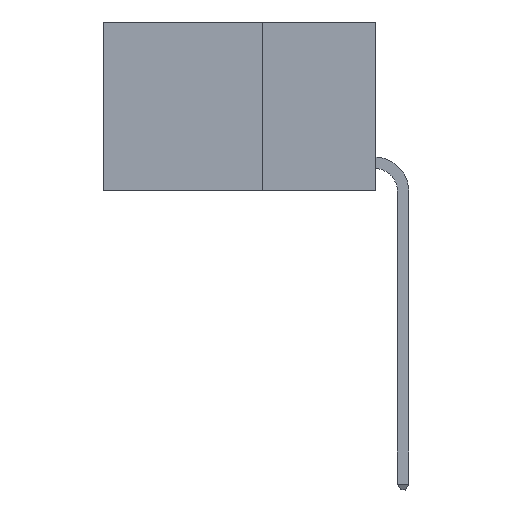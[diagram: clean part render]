
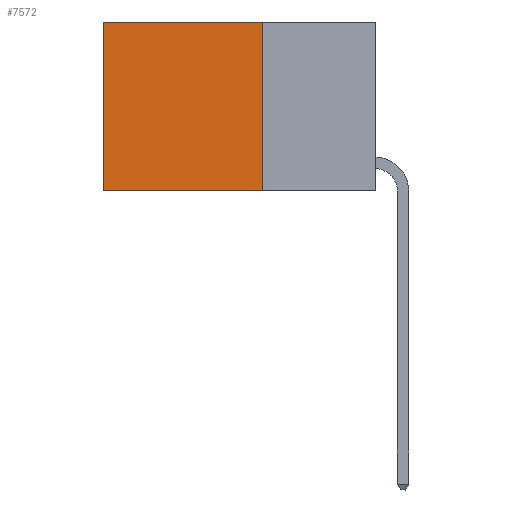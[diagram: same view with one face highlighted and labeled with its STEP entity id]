
A CAD part, left-side view. The second image highlights one B-rep face of the part: STEP entity #7572.
In plain terms, the highlighted planar face has unit normal (-1, 0, 0).
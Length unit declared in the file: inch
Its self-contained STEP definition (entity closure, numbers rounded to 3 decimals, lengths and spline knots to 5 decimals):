
#388 = ORIENTED_EDGE ( 'NONE', *, *, #1872, .F. ) ;
#816 = ORIENTED_EDGE ( 'NONE', *, *, #11375, .F. ) ;
#940 = EDGE_LOOP ( 'NONE', ( #3710, #388, #816, #11710 ) ) ;
#1307 = DIRECTION ( 'NONE',  ( 0., 1., 0. ) ) ;
#1872 = EDGE_CURVE ( 'NONE', #12418, #19040, #2484, .T. ) ;
#2484 = LINE ( 'NONE', #6540, #23468 ) ;
#2777 = VECTOR ( 'NONE', #6769, 39.37008 ) ;
#3455 = VECTOR ( 'NONE', #1307, 39.37008 ) ;
#3710 = ORIENTED_EDGE ( 'NONE', *, *, #16071, .T. ) ;
#3815 = VECTOR ( 'NONE', #17820, 39.37008 ) ;
#3873 = DIRECTION ( 'NONE',  ( 1., 0., 0. ) ) ;
#5211 = AXIS2_PLACEMENT_3D ( 'NONE', #17115, #3873, #11581 ) ;
#5251 = CARTESIAN_POINT ( 'NONE',  ( 0.2625, 0.25, 0. ) ) ;
#5885 = PLANE ( 'NONE',  #5211 ) ;
#6540 = CARTESIAN_POINT ( 'NONE',  ( 0.2625, 0.25, -0.37 ) ) ;
#6769 = DIRECTION ( 'NONE',  ( 0., 0., -1. ) ) ;
#7572 = ADVANCED_FACE ( 'NONE', ( #23262 ), #5885, .F. ) ;
#8710 = VERTEX_POINT ( 'NONE', #22192 ) ;
#8904 = LINE ( 'NONE', #5251, #3455 ) ;
#11375 = EDGE_CURVE ( 'NONE', #8710, #12418, #15661, .T. ) ;
#11581 = DIRECTION ( 'NONE',  ( 0., 0., -1. ) ) ;
#11710 = ORIENTED_EDGE ( 'NONE', *, *, #12006, .T. ) ;
#12006 = EDGE_CURVE ( 'NONE', #8710, #22577, #8904, .T. ) ;
#12418 = VERTEX_POINT ( 'NONE', #16457 ) ;
#14105 = LINE ( 'NONE', #22032, #2777 ) ;
#14255 = DIRECTION ( 'NONE',  ( 0., 1., 0. ) ) ;
#15661 = LINE ( 'NONE', #19825, #3815 ) ;
#16071 = EDGE_CURVE ( 'NONE', #22577, #19040, #14105, .T. ) ;
#16457 = CARTESIAN_POINT ( 'NONE',  ( 0.2625, 0.25, -0.37 ) ) ;
#16869 = CARTESIAN_POINT ( 'NONE',  ( 0.2625, 0.6, -0.37 ) ) ;
#17115 = CARTESIAN_POINT ( 'NONE',  ( 0.2625, 0.25, 0. ) ) ;
#17820 = DIRECTION ( 'NONE',  ( 0., 0., -1. ) ) ;
#18014 = CARTESIAN_POINT ( 'NONE',  ( 0.2625, 0.6, 0. ) ) ;
#19040 = VERTEX_POINT ( 'NONE', #16869 ) ;
#19825 = CARTESIAN_POINT ( 'NONE',  ( 0.2625, 0.25, 0. ) ) ;
#22032 = CARTESIAN_POINT ( 'NONE',  ( 0.2625, 0.6, 0. ) ) ;
#22192 = CARTESIAN_POINT ( 'NONE',  ( 0.2625, 0.25, 0. ) ) ;
#22577 = VERTEX_POINT ( 'NONE', #18014 ) ;
#23262 = FACE_OUTER_BOUND ( 'NONE', #940, .T. ) ;
#23468 = VECTOR ( 'NONE', #14255, 39.37008 ) ;
